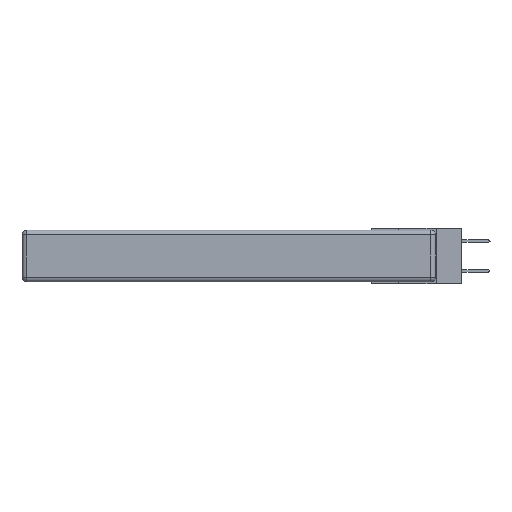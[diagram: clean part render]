
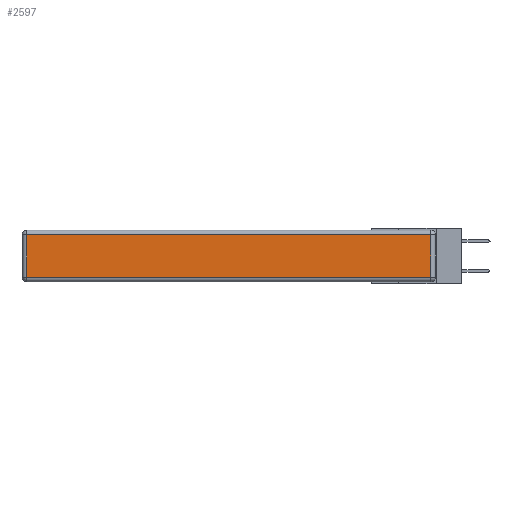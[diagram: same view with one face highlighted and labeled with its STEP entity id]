
A CAD part, left-side view. The second image highlights one B-rep face of the part: STEP entity #2597.
In plain terms, the highlighted planar face has unit normal (-1, 0, 0).
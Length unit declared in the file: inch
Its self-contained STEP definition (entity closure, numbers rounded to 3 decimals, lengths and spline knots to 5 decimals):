
#203 = CARTESIAN_POINT ( 'NONE',  ( 0., 0.03, -0.313 ) ) ;
#600 = DIRECTION ( 'NONE',  ( 0., 0., 1. ) ) ;
#1583 = CARTESIAN_POINT ( 'NONE',  ( 0., 0., -0.343 ) ) ;
#1869 = EDGE_CURVE ( 'NONE', #3501, #2441, #11160, .T. ) ;
#2184 = EDGE_CURVE ( 'NONE', #9636, #10535, #9576, .T. ) ;
#2441 = VERTEX_POINT ( 'NONE', #203 ) ;
#2558 = CARTESIAN_POINT ( 'NONE',  ( 0., 2.72, -0.03 ) ) ;
#2597 = ADVANCED_FACE ( 'NONE', ( #11469 ), #4414, .T. ) ;
#3048 = ORIENTED_EDGE ( 'NONE', *, *, #12387, .T. ) ;
#3058 = CARTESIAN_POINT ( 'NONE',  ( 0., 0.03, -0.343 ) ) ;
#3172 = AXIS2_PLACEMENT_3D ( 'NONE', #1583, #12516, #600 ) ;
#3379 = ORIENTED_EDGE ( 'NONE', *, *, #1869, .T. ) ;
#3494 = CARTESIAN_POINT ( 'NONE',  ( 0., 0.03, -0.03 ) ) ;
#3501 = VERTEX_POINT ( 'NONE', #9871 ) ;
#4099 = VECTOR ( 'NONE', #4807, 39.37008 ) ;
#4267 = VECTOR ( 'NONE', #7696, 39.37008 ) ;
#4414 = PLANE ( 'NONE',  #3172 ) ;
#4768 = EDGE_LOOP ( 'NONE', ( #3379, #3048, #10870, #10928 ) ) ;
#4807 = DIRECTION ( 'NONE',  ( 0., -1., 0. ) ) ;
#5576 = VECTOR ( 'NONE', #12037, 39.37008 ) ;
#5898 = LINE ( 'NONE', #9572, #10577 ) ;
#6541 = DIRECTION ( 'NONE',  ( 0., 0., -1. ) ) ;
#7696 = DIRECTION ( 'NONE',  ( 0., 1., 0. ) ) ;
#9572 = CARTESIAN_POINT ( 'NONE',  ( 0., 2.72, -0.343 ) ) ;
#9576 = LINE ( 'NONE', #12650, #4267 ) ;
#9636 = VERTEX_POINT ( 'NONE', #3494 ) ;
#9871 = CARTESIAN_POINT ( 'NONE',  ( 0., 2.72, -0.313 ) ) ;
#10535 = VERTEX_POINT ( 'NONE', #2558 ) ;
#10577 = VECTOR ( 'NONE', #6541, 39.37008 ) ;
#10870 = ORIENTED_EDGE ( 'NONE', *, *, #2184, .T. ) ;
#10928 = ORIENTED_EDGE ( 'NONE', *, *, #11587, .T. ) ;
#11160 = LINE ( 'NONE', #11559, #4099 ) ;
#11350 = LINE ( 'NONE', #3058, #5576 ) ;
#11469 = FACE_OUTER_BOUND ( 'NONE', #4768, .T. ) ;
#11559 = CARTESIAN_POINT ( 'NONE',  ( 0., 0., -0.313 ) ) ;
#11587 = EDGE_CURVE ( 'NONE', #10535, #3501, #5898, .T. ) ;
#12037 = DIRECTION ( 'NONE',  ( 0., 0., 1. ) ) ;
#12387 = EDGE_CURVE ( 'NONE', #2441, #9636, #11350, .T. ) ;
#12516 = DIRECTION ( 'NONE',  ( -1., 0., 0. ) ) ;
#12650 = CARTESIAN_POINT ( 'NONE',  ( 0., 2.75, -0.03 ) ) ;
